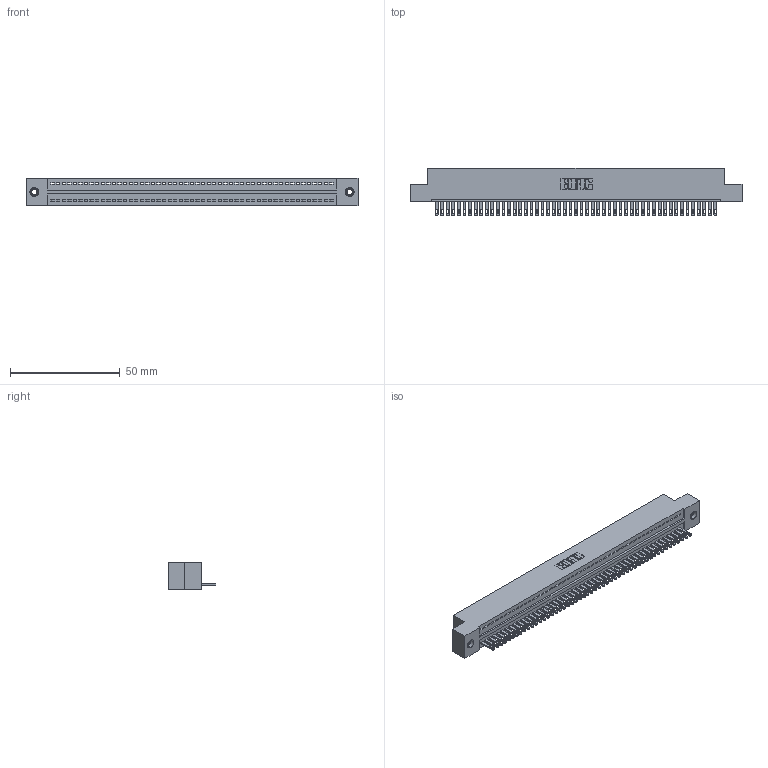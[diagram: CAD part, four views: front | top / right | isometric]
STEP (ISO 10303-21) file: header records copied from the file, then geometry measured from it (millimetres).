
FILE_DESCRIPTION (( 'STEP AP203' ), '1' );
FILE_NAME ('325-051-500-107.STEP', '2020-02-25T00:05:15', ( '' ), ( '' ), 'SwSTEP 2.0', 'SolidWorks 2016', '' );
FILE_SCHEMA (( 'CONFIG_CONTROL_DESIGN' ));
Length unit declared in the file: inch
Products named in the file (4): 325-292-001_325-293-100; 325-051-500-107; 325 Part_TI; 345-250-001_345-250-005-103
Assembly tree (54 placements, depth 2):
  325-051-500-107
    325 Part_TI
    325-292-001_325-293-100  x51
    345-250-001_345-250-005-103  x2
Bounding box: 151.26 x 21.84 x 12.45 mm (x, y, z)
Volume: 19291 mm3; surface area: 21374.7 mm2
Topology: 54 solids, 54 shells, 2928 faces, 9015 edges, 6002 vertices
Faces by surface type: plane 1938, cylinder 974, cone 12, torus 4
Entity records: 31130 total; most frequent: CARTESIAN_POINT 5350, ORIENTED_EDGE 5330, DIRECTION 4529, EDGE_CURVE 2665, LINE 2513, VECTOR 2513, VERTEX_POINT 1772, AXIS2_PLACEMENT_3D 1008
